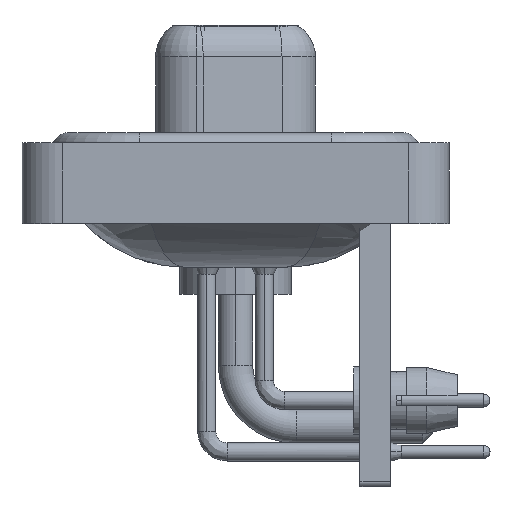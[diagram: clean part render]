
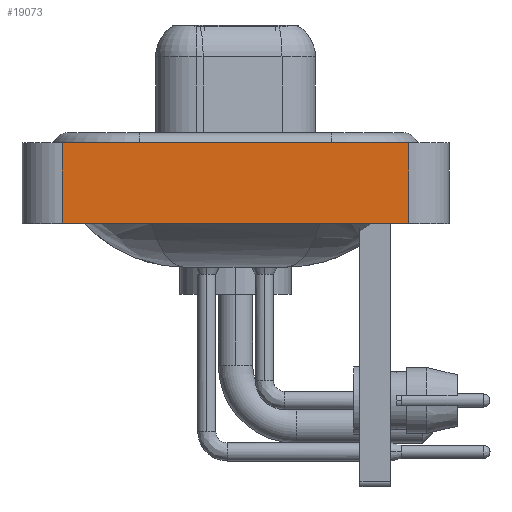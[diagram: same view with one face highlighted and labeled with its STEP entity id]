
A CAD part, left-side view. The second image highlights one B-rep face of the part: STEP entity #19073.
In plain terms, the highlighted planar face has unit normal (-1, 0, 0).
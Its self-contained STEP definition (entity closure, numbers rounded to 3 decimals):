
#72 = VERTEX_POINT ( 'NONE', #21477 ) ;
#1098 = EDGE_CURVE ( 'NONE', #23187, #72, #10776, .T. ) ;
#1429 = EDGE_CURVE ( 'NONE', #72, #24918, #5771, .T. ) ;
#2559 = CARTESIAN_POINT ( 'NONE',  ( -7.35, -8.55, -3.6 ) ) ;
#5616 = ORIENTED_EDGE ( 'NONE', *, *, #1098, .F. ) ;
#5771 = LINE ( 'NONE', #19222, #28811 ) ;
#7379 = CARTESIAN_POINT ( 'NONE',  ( -7.35, -8.55, -3.6 ) ) ;
#7578 = EDGE_CURVE ( 'NONE', #27105, #24918, #10372, .T. ) ;
#10323 = DIRECTION ( 'NONE',  ( 0., -1., 0. ) ) ;
#10372 = LINE ( 'NONE', #7379, #21750 ) ;
#10776 = LINE ( 'NONE', #24101, #14734 ) ;
#10971 = ORIENTED_EDGE ( 'NONE', *, *, #1429, .F. ) ;
#11323 = ORIENTED_EDGE ( 'NONE', *, *, #23174, .T. ) ;
#11925 = FACE_OUTER_BOUND ( 'NONE', #24714, .T. ) ;
#12359 = CARTESIAN_POINT ( 'NONE',  ( -7.35, 8.55, -3.6 ) ) ;
#13952 = DIRECTION ( 'NONE',  ( -1., 0., 0. ) ) ;
#14678 = DIRECTION ( 'NONE',  ( 0., -1., 0. ) ) ;
#14734 = VECTOR ( 'NONE', #19972, 1000. ) ;
#16796 = CARTESIAN_POINT ( 'NONE',  ( -7.35, -8.55, -3.6 ) ) ;
#18628 = PLANE ( 'NONE',  #20674 ) ;
#18932 = CARTESIAN_POINT ( 'NONE',  ( -7.35, -8.55, -3.6 ) ) ;
#19073 = ADVANCED_FACE ( 'NONE', ( #11925 ), #18628, .T. ) ;
#19210 = ORIENTED_EDGE ( 'NONE', *, *, #7578, .T. ) ;
#19222 = CARTESIAN_POINT ( 'NONE',  ( -7.35, -8.55, 0.4 ) ) ;
#19657 = VECTOR ( 'NONE', #10323, 1000. ) ;
#19972 = DIRECTION ( 'NONE',  ( 0., 0., 1. ) ) ;
#20674 = AXIS2_PLACEMENT_3D ( 'NONE', #2559, #13952, #22924 ) ;
#21477 = CARTESIAN_POINT ( 'NONE',  ( -7.35, 8.55, 0.4 ) ) ;
#21750 = VECTOR ( 'NONE', #23193, 1000. ) ;
#22924 = DIRECTION ( 'NONE',  ( 0., 0., 1. ) ) ;
#23045 = CARTESIAN_POINT ( 'NONE',  ( -7.35, -8.55, 0.4 ) ) ;
#23174 = EDGE_CURVE ( 'NONE', #23187, #27105, #23651, .T. ) ;
#23187 = VERTEX_POINT ( 'NONE', #12359 ) ;
#23193 = DIRECTION ( 'NONE',  ( 0., 0., 1. ) ) ;
#23651 = LINE ( 'NONE', #18932, #19657 ) ;
#24101 = CARTESIAN_POINT ( 'NONE',  ( -7.35, 8.55, -3.6 ) ) ;
#24714 = EDGE_LOOP ( 'NONE', ( #19210, #10971, #5616, #11323 ) ) ;
#24918 = VERTEX_POINT ( 'NONE', #23045 ) ;
#27105 = VERTEX_POINT ( 'NONE', #16796 ) ;
#28811 = VECTOR ( 'NONE', #14678, 1000. ) ;
